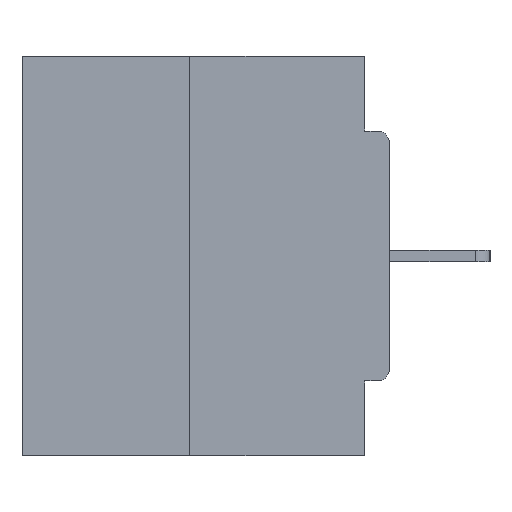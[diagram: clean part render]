
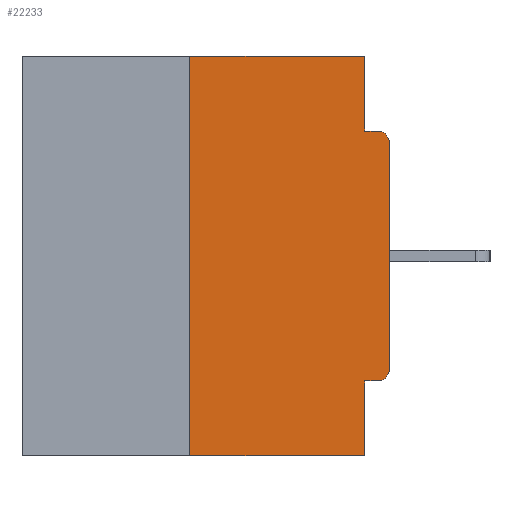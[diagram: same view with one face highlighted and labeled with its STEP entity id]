
A CAD part, left-side view. The second image highlights one B-rep face of the part: STEP entity #22233.
In plain terms, the highlighted planar face has unit normal (-1, 0, 0).
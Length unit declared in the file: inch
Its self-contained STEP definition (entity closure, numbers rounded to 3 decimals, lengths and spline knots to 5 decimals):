
#447 = ORIENTED_EDGE ( 'NONE', *, *, #7671, .F. ) ;
#915 = EDGE_CURVE ( 'NONE', #20354, #17159, #1377, .T. ) ;
#1052 = CARTESIAN_POINT ( 'NONE',  ( 0., 0.031, -0.5 ) ) ;
#1259 = ORIENTED_EDGE ( 'NONE', *, *, #915, .F. ) ;
#1313 = DIRECTION ( 'NONE',  ( 0., 0., -1. ) ) ;
#1377 = LINE ( 'NONE', #1052, #9214 ) ;
#1449 = ORIENTED_EDGE ( 'NONE', *, *, #33338, .T. ) ;
#1509 = ORIENTED_EDGE ( 'NONE', *, *, #13968, .F. ) ;
#1658 = VECTOR ( 'NONE', #12963, 39.37008 ) ;
#1693 = VERTEX_POINT ( 'NONE', #12357 ) ;
#1774 = CARTESIAN_POINT ( 'NONE',  ( 0., 0., -0.3915 ) ) ;
#1968 = ORIENTED_EDGE ( 'NONE', *, *, #30521, .F. ) ;
#2274 = CARTESIAN_POINT ( 'NONE',  ( 0., 0.25, -0.5 ) ) ;
#2937 = CARTESIAN_POINT ( 'NONE',  ( 0., 0., -0.0935 ) ) ;
#3676 = ORIENTED_EDGE ( 'NONE', *, *, #31162, .T. ) ;
#4463 = PLANE ( 'NONE',  #25809 ) ;
#4630 = EDGE_CURVE ( 'NONE', #7399, #18217, #29212, .T. ) ;
#5114 = CARTESIAN_POINT ( 'NONE',  ( 0., 0.25, 0. ) ) ;
#7094 = DIRECTION ( 'NONE',  ( 0., 0., -1. ) ) ;
#7139 = CARTESIAN_POINT ( 'NONE',  ( 0., 0.031, -0.5 ) ) ;
#7399 = VERTEX_POINT ( 'NONE', #1774 ) ;
#7614 = LINE ( 'NONE', #15298, #13704 ) ;
#7671 = EDGE_CURVE ( 'NONE', #1693, #20354, #11344, .T. ) ;
#7955 = VERTEX_POINT ( 'NONE', #32123 ) ;
#8421 = VERTEX_POINT ( 'NONE', #2274 ) ;
#8540 = VECTOR ( 'NONE', #17227, 39.37008 ) ;
#8716 = AXIS2_PLACEMENT_3D ( 'NONE', #25127, #9671, #27696 ) ;
#9214 = VECTOR ( 'NONE', #1313, 39.37008 ) ;
#9625 = ORIENTED_EDGE ( 'NONE', *, *, #13305, .F. ) ;
#9671 = DIRECTION ( 'NONE',  ( -1., 0., 0. ) ) ;
#9865 = EDGE_LOOP ( 'NONE', ( #1968, #1509, #1449, #1259, #447, #3676, #12265, #19469, #16536, #9625 ) ) ;
#10814 = DIRECTION ( 'NONE',  ( 0., -1., 0. ) ) ;
#10918 = LINE ( 'NONE', #19111, #30602 ) ;
#11344 = LINE ( 'NONE', #17320, #23496 ) ;
#12265 = ORIENTED_EDGE ( 'NONE', *, *, #4630, .T. ) ;
#12357 = CARTESIAN_POINT ( 'NONE',  ( 0., 0.015, -0.4065 ) ) ;
#12799 = DIRECTION ( 'NONE',  ( -1., 0., 0. ) ) ;
#12963 = DIRECTION ( 'NONE',  ( 0., 0., 1. ) ) ;
#13181 = CARTESIAN_POINT ( 'NONE',  ( 0., 0., 0. ) ) ;
#13305 = EDGE_CURVE ( 'NONE', #28749, #7955, #21847, .T. ) ;
#13704 = VECTOR ( 'NONE', #30641, 39.37008 ) ;
#13968 = EDGE_CURVE ( 'NONE', #8421, #16676, #7614, .T. ) ;
#14273 = CIRCLE ( 'NONE', #8716, 0.015 ) ;
#14942 = VECTOR ( 'NONE', #27915, 39.37008 ) ;
#15030 = VERTEX_POINT ( 'NONE', #30347 ) ;
#15298 = CARTESIAN_POINT ( 'NONE',  ( 0., 0.25, 0. ) ) ;
#16536 = ORIENTED_EDGE ( 'NONE', *, *, #28785, .F. ) ;
#16676 = VERTEX_POINT ( 'NONE', #5114 ) ;
#17124 = DIRECTION ( 'NONE',  ( 0., 1., 0. ) ) ;
#17159 = VERTEX_POINT ( 'NONE', #7139 ) ;
#17227 = DIRECTION ( 'NONE',  ( 0., -1., 0. ) ) ;
#17320 = CARTESIAN_POINT ( 'NONE',  ( 0., 0., -0.4065 ) ) ;
#17724 = CARTESIAN_POINT ( 'NONE',  ( 0., 0.031, 0. ) ) ;
#18217 = VERTEX_POINT ( 'NONE', #32975 ) ;
#19111 = CARTESIAN_POINT ( 'NONE',  ( 0., 0.46, -0.5 ) ) ;
#19469 = ORIENTED_EDGE ( 'NONE', *, *, #29928, .T. ) ;
#20354 = VERTEX_POINT ( 'NONE', #21744 ) ;
#21744 = CARTESIAN_POINT ( 'NONE',  ( 0., 0.031, -0.4065 ) ) ;
#21847 = LINE ( 'NONE', #17724, #14942 ) ;
#22233 = ADVANCED_FACE ( 'NONE', ( #23840 ), #4463, .F. ) ;
#22334 = CARTESIAN_POINT ( 'NONE',  ( 0., 0.46, 0. ) ) ;
#22338 = LINE ( 'NONE', #22334, #8540 ) ;
#22599 = DIRECTION ( 'NONE',  ( 1., 0., 0. ) ) ;
#23496 = VECTOR ( 'NONE', #17124, 39.37008 ) ;
#23840 = FACE_OUTER_BOUND ( 'NONE', #9865, .T. ) ;
#24053 = VECTOR ( 'NONE', #10814, 39.37008 ) ;
#24263 = CIRCLE ( 'NONE', #28611, 0.015 ) ;
#25019 = CARTESIAN_POINT ( 'NONE',  ( 0., 0.46, 0. ) ) ;
#25127 = CARTESIAN_POINT ( 'NONE',  ( 0., 0.015, -0.1085 ) ) ;
#25809 = AXIS2_PLACEMENT_3D ( 'NONE', #25019, #22599, #7094 ) ;
#26026 = CARTESIAN_POINT ( 'NONE',  ( 0., 0.031, 0. ) ) ;
#27696 = DIRECTION ( 'NONE',  ( 0., 0., -1. ) ) ;
#27915 = DIRECTION ( 'NONE',  ( 0., 0., -1. ) ) ;
#28193 = CARTESIAN_POINT ( 'NONE',  ( 0., 0.015, -0.3915 ) ) ;
#28611 = AXIS2_PLACEMENT_3D ( 'NONE', #28193, #12799, #30736 ) ;
#28749 = VERTEX_POINT ( 'NONE', #26026 ) ;
#28785 = EDGE_CURVE ( 'NONE', #7955, #15030, #31605, .T. ) ;
#29212 = LINE ( 'NONE', #13181, #1658 ) ;
#29282 = DIRECTION ( 'NONE',  ( 0., -1., 0. ) ) ;
#29928 = EDGE_CURVE ( 'NONE', #18217, #15030, #14273, .T. ) ;
#30347 = CARTESIAN_POINT ( 'NONE',  ( 0., 0.015, -0.0935 ) ) ;
#30521 = EDGE_CURVE ( 'NONE', #16676, #28749, #22338, .T. ) ;
#30602 = VECTOR ( 'NONE', #29282, 39.37008 ) ;
#30641 = DIRECTION ( 'NONE',  ( 0., 0., 1. ) ) ;
#30736 = DIRECTION ( 'NONE',  ( 0., 0., -1. ) ) ;
#31162 = EDGE_CURVE ( 'NONE', #1693, #7399, #24263, .T. ) ;
#31605 = LINE ( 'NONE', #2937, #24053 ) ;
#32123 = CARTESIAN_POINT ( 'NONE',  ( 0., 0.031, -0.0935 ) ) ;
#32975 = CARTESIAN_POINT ( 'NONE',  ( 0., 0., -0.1085 ) ) ;
#33338 = EDGE_CURVE ( 'NONE', #8421, #17159, #10918, .T. ) ;
